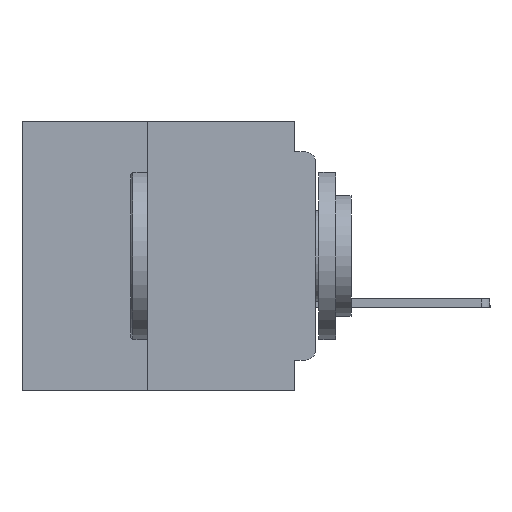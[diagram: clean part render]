
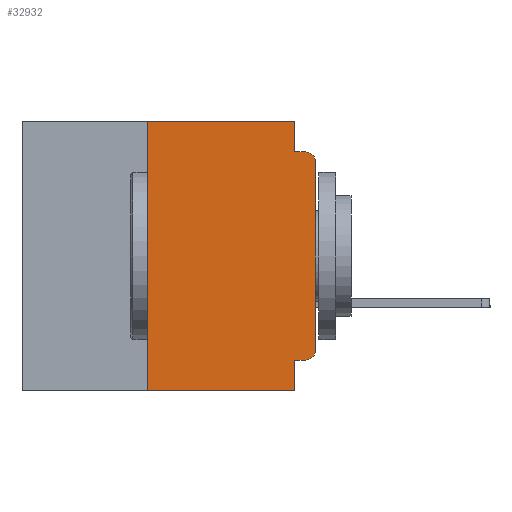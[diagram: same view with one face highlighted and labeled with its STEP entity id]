
A CAD part, left-side view. The second image highlights one B-rep face of the part: STEP entity #32932.
In plain terms, the highlighted planar face has unit normal (-1, 0, 0).
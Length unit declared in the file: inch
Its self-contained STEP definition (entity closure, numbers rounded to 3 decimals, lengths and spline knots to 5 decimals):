
#1198 = VERTEX_POINT ( 'NONE', #28562 ) ;
#1424 = EDGE_CURVE ( 'NONE', #42169, #45362, #42618, .T. ) ;
#3295 = EDGE_CURVE ( 'NONE', #44852, #5277, #28555, .T. ) ;
#3731 = CARTESIAN_POINT ( 'NONE',  ( 0., 0.015, -0.045 ) ) ;
#5253 = VECTOR ( 'NONE', #13754, 39.37008 ) ;
#5277 = VERTEX_POINT ( 'NONE', #3731 ) ;
#5709 = DIRECTION ( 'NONE',  ( 0., 0., -1. ) ) ;
#5973 = DIRECTION ( 'NONE',  ( -1., 0., 0. ) ) ;
#6093 = CARTESIAN_POINT ( 'NONE',  ( 0., 0.031, -0.4 ) ) ;
#6305 = VERTEX_POINT ( 'NONE', #44161 ) ;
#6342 = CARTESIAN_POINT ( 'NONE',  ( 0., 0.015, -0.06 ) ) ;
#7063 = DIRECTION ( 'NONE',  ( -1., 0., 0. ) ) ;
#7890 = DIRECTION ( 'NONE',  ( 0., 0., 1. ) ) ;
#8529 = CARTESIAN_POINT ( 'NONE',  ( 0., 0.437, 0. ) ) ;
#8676 = PLANE ( 'NONE',  #29268 ) ;
#8703 = EDGE_CURVE ( 'NONE', #1198, #6305, #37291, .T. ) ;
#11067 = DIRECTION ( 'NONE',  ( 0., -1., 0. ) ) ;
#11229 = CARTESIAN_POINT ( 'NONE',  ( 0., 0.437, 0. ) ) ;
#12215 = CARTESIAN_POINT ( 'NONE',  ( 0., 0.25, -0.4 ) ) ;
#12284 = DIRECTION ( 'NONE',  ( 0., 0., -1. ) ) ;
#12631 = ORIENTED_EDGE ( 'NONE', *, *, #44904, .T. ) ;
#12974 = EDGE_LOOP ( 'NONE', ( #25942, #36285, #37827, #38367, #30462, #24913, #16567, #38468, #46152, #12631 ) ) ;
#13037 = VECTOR ( 'NONE', #38282, 39.37008 ) ;
#13637 = DIRECTION ( 'NONE',  ( 0., 1., 0. ) ) ;
#13754 = DIRECTION ( 'NONE',  ( 0., -1., 0. ) ) ;
#14462 = VECTOR ( 'NONE', #13637, 39.37008 ) ;
#15355 = EDGE_CURVE ( 'NONE', #19868, #29399, #41745, .T. ) ;
#16210 = VECTOR ( 'NONE', #41023, 39.37008 ) ;
#16567 = ORIENTED_EDGE ( 'NONE', *, *, #45438, .T. ) ;
#17267 = CARTESIAN_POINT ( 'NONE',  ( 0., 0.015, -0.355 ) ) ;
#17278 = VERTEX_POINT ( 'NONE', #28268 ) ;
#17848 = CARTESIAN_POINT ( 'NONE',  ( 0., 0.031, -0.355 ) ) ;
#19225 = EDGE_CURVE ( 'NONE', #43826, #44852, #25896, .T. ) ;
#19868 = VERTEX_POINT ( 'NONE', #17267 ) ;
#20310 = CARTESIAN_POINT ( 'NONE',  ( 0., 0.25, 0. ) ) ;
#23682 = VECTOR ( 'NONE', #7890, 39.37008 ) ;
#24227 = CARTESIAN_POINT ( 'NONE',  ( 0., 0., -0.355 ) ) ;
#24817 = FACE_OUTER_BOUND ( 'NONE', #12974, .T. ) ;
#24913 = ORIENTED_EDGE ( 'NONE', *, *, #1424, .F. ) ;
#25518 = AXIS2_PLACEMENT_3D ( 'NONE', #28465, #7063, #32040 ) ;
#25896 = LINE ( 'NONE', #41309, #35410 ) ;
#25942 = ORIENTED_EDGE ( 'NONE', *, *, #19225, .T. ) ;
#28268 = CARTESIAN_POINT ( 'NONE',  ( 0., 0.031, -0.4 ) ) ;
#28465 = CARTESIAN_POINT ( 'NONE',  ( 0., 0.015, -0.34 ) ) ;
#28555 = CIRCLE ( 'NONE', #38004, 0.015 ) ;
#28562 = CARTESIAN_POINT ( 'NONE',  ( 0., 0.031, 0. ) ) ;
#28806 = CIRCLE ( 'NONE', #25518, 0.015 ) ;
#29268 = AXIS2_PLACEMENT_3D ( 'NONE', #8529, #33682, #12284 ) ;
#29392 = LINE ( 'NONE', #11229, #39990 ) ;
#29399 = VERTEX_POINT ( 'NONE', #17848 ) ;
#29698 = EDGE_CURVE ( 'NONE', #6305, #5277, #44667, .T. ) ;
#29904 = CARTESIAN_POINT ( 'NONE',  ( 0., 0.031, 0. ) ) ;
#30000 = DIRECTION ( 'NONE',  ( 0., 0., -1. ) ) ;
#30462 = ORIENTED_EDGE ( 'NONE', *, *, #31913, .F. ) ;
#31719 = CARTESIAN_POINT ( 'NONE',  ( 0., 0., -0.06 ) ) ;
#31913 = EDGE_CURVE ( 'NONE', #45362, #1198, #29392, .T. ) ;
#32040 = DIRECTION ( 'NONE',  ( 0., 0., -1. ) ) ;
#32932 = ADVANCED_FACE ( 'NONE', ( #24817 ), #8676, .F. ) ;
#33682 = DIRECTION ( 'NONE',  ( 1., 0., 0. ) ) ;
#33791 = LINE ( 'NONE', #35155, #5253 ) ;
#35155 = CARTESIAN_POINT ( 'NONE',  ( 0., 0.437, -0.4 ) ) ;
#35410 = VECTOR ( 'NONE', #44899, 39.37008 ) ;
#35824 = CARTESIAN_POINT ( 'NONE',  ( 0., 0.25, -0.4 ) ) ;
#36196 = VECTOR ( 'NONE', #30000, 39.37008 ) ;
#36285 = ORIENTED_EDGE ( 'NONE', *, *, #3295, .T. ) ;
#36401 = CARTESIAN_POINT ( 'NONE',  ( 0., 0., -0.34 ) ) ;
#37291 = LINE ( 'NONE', #29904, #36196 ) ;
#37827 = ORIENTED_EDGE ( 'NONE', *, *, #29698, .F. ) ;
#38004 = AXIS2_PLACEMENT_3D ( 'NONE', #6342, #5973, #5709 ) ;
#38282 = DIRECTION ( 'NONE',  ( 0., 0., -1. ) ) ;
#38337 = EDGE_CURVE ( 'NONE', #29399, #17278, #41439, .T. ) ;
#38367 = ORIENTED_EDGE ( 'NONE', *, *, #8703, .F. ) ;
#38468 = ORIENTED_EDGE ( 'NONE', *, *, #38337, .F. ) ;
#39990 = VECTOR ( 'NONE', #11067, 39.37008 ) ;
#41023 = DIRECTION ( 'NONE',  ( 0., -1., 0. ) ) ;
#41309 = CARTESIAN_POINT ( 'NONE',  ( 0., 0., 0. ) ) ;
#41439 = LINE ( 'NONE', #6093, #13037 ) ;
#41745 = LINE ( 'NONE', #24227, #14462 ) ;
#42169 = VERTEX_POINT ( 'NONE', #12215 ) ;
#42618 = LINE ( 'NONE', #35824, #23682 ) ;
#43826 = VERTEX_POINT ( 'NONE', #36401 ) ;
#44161 = CARTESIAN_POINT ( 'NONE',  ( 0., 0.031, -0.045 ) ) ;
#44616 = CARTESIAN_POINT ( 'NONE',  ( 0., 0., -0.045 ) ) ;
#44667 = LINE ( 'NONE', #44616, #16210 ) ;
#44852 = VERTEX_POINT ( 'NONE', #31719 ) ;
#44899 = DIRECTION ( 'NONE',  ( 0., 0., 1. ) ) ;
#44904 = EDGE_CURVE ( 'NONE', #19868, #43826, #28806, .T. ) ;
#45362 = VERTEX_POINT ( 'NONE', #20310 ) ;
#45438 = EDGE_CURVE ( 'NONE', #42169, #17278, #33791, .T. ) ;
#46152 = ORIENTED_EDGE ( 'NONE', *, *, #15355, .F. ) ;
